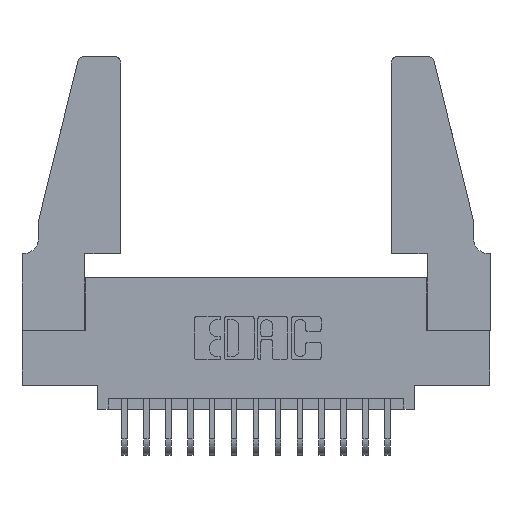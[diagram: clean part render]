
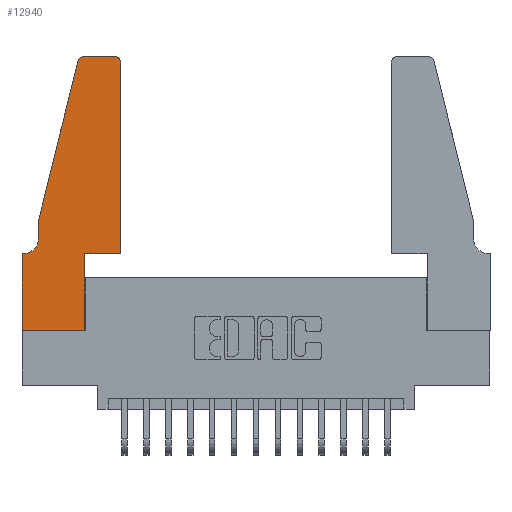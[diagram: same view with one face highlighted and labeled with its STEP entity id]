
A CAD part, top view. The second image highlights one B-rep face of the part: STEP entity #12940.
In plain terms, the highlighted planar face has unit normal (0, 0, 1).
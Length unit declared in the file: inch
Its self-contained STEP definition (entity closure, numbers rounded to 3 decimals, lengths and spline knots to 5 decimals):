
#275 = AXIS2_PLACEMENT_3D ( 'NONE', #15724, #7396, #17090 ) ;
#322 = ORIENTED_EDGE ( 'NONE', *, *, #7895, .T. ) ;
#690 = VERTEX_POINT ( 'NONE', #13412 ) ;
#791 = CARTESIAN_POINT ( 'NONE',  ( 0.284, 1.22, 0.37 ) ) ;
#830 = AXIS2_PLACEMENT_3D ( 'NONE', #4097, #13900, #5520 ) ;
#1037 = ORIENTED_EDGE ( 'NONE', *, *, #7073, .T. ) ;
#1307 = CARTESIAN_POINT ( 'NONE',  ( 0.0755, 0.42, 0.37 ) ) ;
#1317 = LINE ( 'NONE', #12798, #15726 ) ;
#1459 = ORIENTED_EDGE ( 'NONE', *, *, #9828, .T. ) ;
#1563 = EDGE_CURVE ( 'NONE', #9839, #17272, #2906, .T. ) ;
#1628 = CARTESIAN_POINT ( 'NONE',  ( 0., 0.35, 0.37 ) ) ;
#1789 = AXIS2_PLACEMENT_3D ( 'NONE', #791, #10608, #2186 ) ;
#1899 = VECTOR ( 'NONE', #17513, 39.37008 ) ;
#2155 = VERTEX_POINT ( 'NONE', #4733 ) ;
#2186 = DIRECTION ( 'NONE',  ( 1., 0., 0. ) ) ;
#2455 = VERTEX_POINT ( 'NONE', #1307 ) ;
#2477 = VECTOR ( 'NONE', #17693, 39.37008 ) ;
#2767 = ORIENTED_EDGE ( 'NONE', *, *, #3381, .T. ) ;
#2881 = EDGE_CURVE ( 'NONE', #11332, #16773, #15747, .T. ) ;
#2906 = LINE ( 'NONE', #15857, #14085 ) ;
#3036 = PLANE ( 'NONE',  #17444 ) ;
#3262 = EDGE_CURVE ( 'NONE', #17272, #2455, #1317, .T. ) ;
#3350 = CARTESIAN_POINT ( 'NONE',  ( 0.0755, 0.35, 0.37 ) ) ;
#3381 = EDGE_CURVE ( 'NONE', #2155, #9694, #17219, .T. ) ;
#3400 = VERTEX_POINT ( 'NONE', #15739 ) ;
#4082 = VERTEX_POINT ( 'NONE', #4671 ) ;
#4097 = CARTESIAN_POINT ( 'NONE',  ( 0.4205, 1.22, 0.37 ) ) ;
#4150 = LINE ( 'NONE', #12696, #14447 ) ;
#4172 = VECTOR ( 'NONE', #11949, 39.37008 ) ;
#4439 = DIRECTION ( 'NONE',  ( 1., 0., 0. ) ) ;
#4579 = DIRECTION ( 'NONE',  ( 0., 1., 0. ) ) ;
#4671 = CARTESIAN_POINT ( 'NONE',  ( 0.0055, 0.35, 0.37 ) ) ;
#4733 = CARTESIAN_POINT ( 'NONE',  ( 0.4505, 0.35, 0.37 ) ) ;
#5147 = CIRCLE ( 'NONE', #830, 0.03 ) ;
#5520 = DIRECTION ( 'NONE',  ( 1., 0., 0. ) ) ;
#5708 = DIRECTION ( 'NONE',  ( 1., 0., 0. ) ) ;
#6002 = CARTESIAN_POINT ( 'NONE',  ( 0.4505, 0.35, 0.37 ) ) ;
#6157 = CARTESIAN_POINT ( 'NONE',  ( 0.284, 1.25, 0.37 ) ) ;
#6346 = EDGE_CURVE ( 'NONE', #690, #3400, #11372, .T. ) ;
#7073 = EDGE_CURVE ( 'NONE', #4082, #690, #17590, .T. ) ;
#7396 = DIRECTION ( 'NONE',  ( 0., 0., -1. ) ) ;
#7516 = DIRECTION ( 'NONE',  ( -0.239, -0.971, 0. ) ) ;
#7642 = VECTOR ( 'NONE', #10315, 39.37008 ) ;
#7806 = CARTESIAN_POINT ( 'NONE',  ( 0.2605, 1.25, 0.37 ) ) ;
#7895 = EDGE_CURVE ( 'NONE', #9761, #10359, #12206, .T. ) ;
#8151 = CIRCLE ( 'NONE', #1789, 0.03 ) ;
#8674 = ORIENTED_EDGE ( 'NONE', *, *, #3262, .T. ) ;
#8789 = EDGE_CURVE ( 'NONE', #9694, #9761, #5147, .T. ) ;
#9216 = CARTESIAN_POINT ( 'NONE',  ( 0.2865, 0., 0.37 ) ) ;
#9335 = ORIENTED_EDGE ( 'NONE', *, *, #10664, .T. ) ;
#9353 = ORIENTED_EDGE ( 'NONE', *, *, #12224, .T. ) ;
#9423 = CIRCLE ( 'NONE', #275, 0.07 ) ;
#9694 = VERTEX_POINT ( 'NONE', #17284 ) ;
#9761 = VERTEX_POINT ( 'NONE', #11978 ) ;
#9828 = EDGE_CURVE ( 'NONE', #3400, #11332, #9948, .T. ) ;
#9839 = VERTEX_POINT ( 'NONE', #14999 ) ;
#9861 = FACE_OUTER_BOUND ( 'NONE', #15976, .T. ) ;
#9948 = LINE ( 'NONE', #10822, #2477 ) ;
#10315 = DIRECTION ( 'NONE',  ( 0., -1., 0. ) ) ;
#10352 = CARTESIAN_POINT ( 'NONE',  ( 0.2865, 0.35, 0.37 ) ) ;
#10359 = VERTEX_POINT ( 'NONE', #6157 ) ;
#10465 = ORIENTED_EDGE ( 'NONE', *, *, #13001, .T. ) ;
#10608 = DIRECTION ( 'NONE',  ( 0., 0., 1. ) ) ;
#10664 = EDGE_CURVE ( 'NONE', #10359, #9839, #8151, .T. ) ;
#10822 = CARTESIAN_POINT ( 'NONE',  ( 0., 0., 0.37 ) ) ;
#11332 = VERTEX_POINT ( 'NONE', #9216 ) ;
#11372 = LINE ( 'NONE', #14449, #7642 ) ;
#11538 = ORIENTED_EDGE ( 'NONE', *, *, #1563, .T. ) ;
#11746 = DIRECTION ( 'NONE',  ( -1., 0., 0. ) ) ;
#11949 = DIRECTION ( 'NONE',  ( 0., 1., 0. ) ) ;
#11978 = CARTESIAN_POINT ( 'NONE',  ( 0.4205, 1.25, 0.37 ) ) ;
#12198 = ORIENTED_EDGE ( 'NONE', *, *, #6346, .T. ) ;
#12206 = LINE ( 'NONE', #7806, #1899 ) ;
#12224 = EDGE_CURVE ( 'NONE', #16773, #2155, #4150, .T. ) ;
#12696 = CARTESIAN_POINT ( 'NONE',  ( 0.4505, 0.35, 0.37 ) ) ;
#12798 = CARTESIAN_POINT ( 'NONE',  ( 0.0755, 0.5, 0.37 ) ) ;
#12838 = DIRECTION ( 'NONE',  ( 0., 0., 1. ) ) ;
#12940 = ADVANCED_FACE ( 'NONE', ( #9861 ), #3036, .T. ) ;
#13001 = EDGE_CURVE ( 'NONE', #2455, #4082, #9423, .T. ) ;
#13412 = CARTESIAN_POINT ( 'NONE',  ( 0., 0.35, 0.37 ) ) ;
#13900 = DIRECTION ( 'NONE',  ( 0., 0., 1. ) ) ;
#13962 = VECTOR ( 'NONE', #11746, 39.37008 ) ;
#14021 = VECTOR ( 'NONE', #4579, 39.37008 ) ;
#14085 = VECTOR ( 'NONE', #7516, 39.37008 ) ;
#14199 = DIRECTION ( 'NONE',  ( 0., -1., 0. ) ) ;
#14286 = CARTESIAN_POINT ( 'NONE',  ( 0.0755, 0.5, 0.37 ) ) ;
#14447 = VECTOR ( 'NONE', #5708, 39.37008 ) ;
#14449 = CARTESIAN_POINT ( 'NONE',  ( 0., 0., 0.37 ) ) ;
#14999 = CARTESIAN_POINT ( 'NONE',  ( 0.25487, 1.22718, 0.37 ) ) ;
#15724 = CARTESIAN_POINT ( 'NONE',  ( 0.0055, 0.42, 0.37 ) ) ;
#15726 = VECTOR ( 'NONE', #14199, 39.37008 ) ;
#15739 = CARTESIAN_POINT ( 'NONE',  ( 0., 0., 0.37 ) ) ;
#15747 = LINE ( 'NONE', #17542, #4172 ) ;
#15857 = CARTESIAN_POINT ( 'NONE',  ( 0.0755, 0.5, 0.37 ) ) ;
#15976 = EDGE_LOOP ( 'NONE', ( #322, #9335, #11538, #8674, #10465, #1037, #12198, #1459, #16293, #9353, #2767, #18016 ) ) ;
#16293 = ORIENTED_EDGE ( 'NONE', *, *, #2881, .T. ) ;
#16773 = VERTEX_POINT ( 'NONE', #10352 ) ;
#17090 = DIRECTION ( 'NONE',  ( -1., 0., 0. ) ) ;
#17219 = LINE ( 'NONE', #6002, #14021 ) ;
#17272 = VERTEX_POINT ( 'NONE', #14286 ) ;
#17284 = CARTESIAN_POINT ( 'NONE',  ( 0.4505, 1.22, 0.37 ) ) ;
#17444 = AXIS2_PLACEMENT_3D ( 'NONE', #1628, #12838, #4439 ) ;
#17513 = DIRECTION ( 'NONE',  ( -1., 0., 0. ) ) ;
#17542 = CARTESIAN_POINT ( 'NONE',  ( 0.2865, 0.35, 0.37 ) ) ;
#17590 = LINE ( 'NONE', #3350, #13962 ) ;
#17693 = DIRECTION ( 'NONE',  ( 1., 0., 0. ) ) ;
#18016 = ORIENTED_EDGE ( 'NONE', *, *, #8789, .T. ) ;
